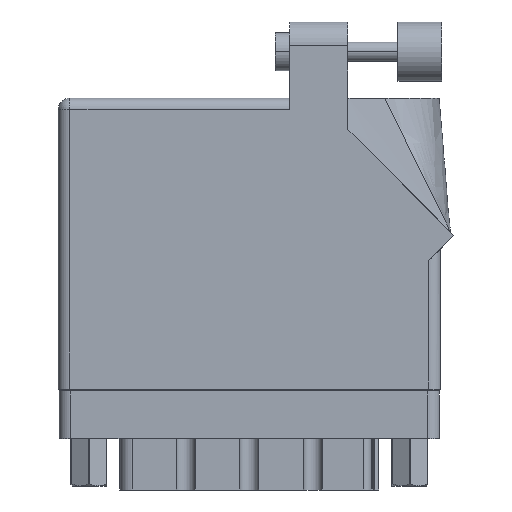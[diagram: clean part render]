
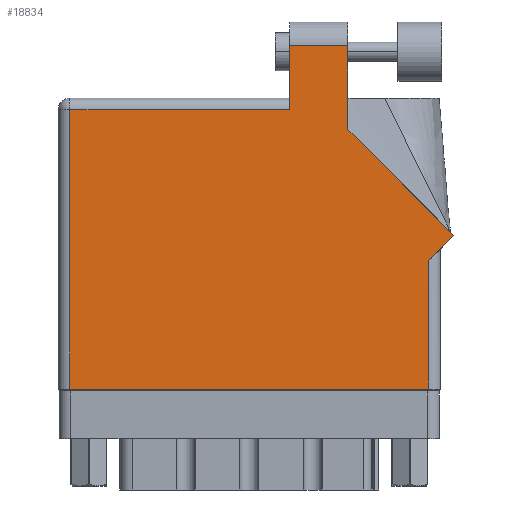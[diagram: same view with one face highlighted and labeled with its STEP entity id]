
A CAD part, front view. The second image highlights one B-rep face of the part: STEP entity #18834.
In plain terms, the highlighted face is planar.
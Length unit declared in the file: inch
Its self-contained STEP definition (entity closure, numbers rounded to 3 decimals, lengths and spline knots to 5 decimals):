
#185 = CARTESIAN_POINT ( 'NONE',  ( 0.062, 1.468, 0. ) ) ;
#529 = CARTESIAN_POINT ( 'NONE',  ( 1.524, 1.36442, 0. ) ) ;
#2475 = EDGE_CURVE ( 'NONE', #21599, #13160, #9164, .T. ) ;
#2711 = DIRECTION ( 'NONE',  ( 0., -1., 0. ) ) ;
#2892 = LINE ( 'NONE', #22346, #11988 ) ;
#3526 = CARTESIAN_POINT ( 'NONE',  ( 0.062, 0., 0. ) ) ;
#4853 = ORIENTED_EDGE ( 'NONE', *, *, #49832, .T. ) ;
#5081 = LINE ( 'NONE', #19882, #40089 ) ;
#5888 = CARTESIAN_POINT ( 'NONE',  ( 1.948, 0., 0. ) ) ;
#7686 = DIRECTION ( 'NONE',  ( 0., 0., -1. ) ) ;
#7887 = CARTESIAN_POINT ( 'NONE',  ( 1.948, 0.737, 0. ) ) ;
#7978 = VERTEX_POINT ( 'NONE', #42189 ) ;
#8332 = ORIENTED_EDGE ( 'NONE', *, *, #29546, .T. ) ;
#9164 = LINE ( 'NONE', #31423, #41724 ) ;
#9362 = LINE ( 'NONE', #35541, #27454 ) ;
#10418 = AXIS2_PLACEMENT_3D ( 'NONE', #46684, #7686, #23366 ) ;
#11100 = ORIENTED_EDGE ( 'NONE', *, *, #23640, .T. ) ;
#11988 = VECTOR ( 'NONE', #2711, 39.37008 ) ;
#12071 = DIRECTION ( 'NONE',  ( 0., -1., 0. ) ) ;
#12095 = CARTESIAN_POINT ( 'NONE',  ( 1.217, 1.805, 0. ) ) ;
#12140 = DIRECTION ( 'NONE',  ( 0.707, 0.707, 0. ) ) ;
#12303 = DIRECTION ( 'NONE',  ( 0., 1., 0. ) ) ;
#13160 = VERTEX_POINT ( 'NONE', #3526 ) ;
#13547 = ORIENTED_EDGE ( 'NONE', *, *, #33288, .T. ) ;
#13763 = VECTOR ( 'NONE', #20716, 39.37008 ) ;
#14477 = VERTEX_POINT ( 'NONE', #38979 ) ;
#14538 = FACE_OUTER_BOUND ( 'NONE', #25998, .T. ) ;
#14800 = VERTEX_POINT ( 'NONE', #25847 ) ;
#16198 = ORIENTED_EDGE ( 'NONE', *, *, #37717, .T. ) ;
#16261 = LINE ( 'NONE', #12095, #19901 ) ;
#18834 = ADVANCED_FACE ( 'NONE', ( #14538 ), #42511, .F. ) ;
#18990 = CARTESIAN_POINT ( 'NONE',  ( 2.08071, 0.80771, 0. ) ) ;
#19057 = DIRECTION ( 'NONE',  ( -1., 0., 0. ) ) ;
#19882 = CARTESIAN_POINT ( 'NONE',  ( 0., 1.468, 0. ) ) ;
#19901 = VECTOR ( 'NONE', #19057, 39.37008 ) ;
#20716 = DIRECTION ( 'NONE',  ( 0., 1., 0. ) ) ;
#21599 = VERTEX_POINT ( 'NONE', #185 ) ;
#22231 = LINE ( 'NONE', #44333, #13763 ) ;
#22346 = CARTESIAN_POINT ( 'NONE',  ( 1.217, 1.53, 0. ) ) ;
#23366 = DIRECTION ( 'NONE',  ( -1., 0., 0. ) ) ;
#23640 = EDGE_CURVE ( 'NONE', #33183, #21599, #5081, .T. ) ;
#23658 = ORIENTED_EDGE ( 'NONE', *, *, #2475, .T. ) ;
#23782 = DIRECTION ( 'NONE',  ( 1., 0., 0. ) ) ;
#24541 = LINE ( 'NONE', #18990, #48590 ) ;
#25847 = CARTESIAN_POINT ( 'NONE',  ( 1.524, 1.805, 0. ) ) ;
#25998 = EDGE_LOOP ( 'NONE', ( #4853, #31379, #16198, #11100, #23658, #13547, #8332, #40610, #35403 ) ) ;
#26189 = VECTOR ( 'NONE', #12303, 39.37008 ) ;
#26831 = CARTESIAN_POINT ( 'NONE',  ( 1.217, 1.468, 0. ) ) ;
#27454 = VECTOR ( 'NONE', #12140, 39.37008 ) ;
#27511 = EDGE_CURVE ( 'NONE', #14477, #28254, #24541, .T. ) ;
#27659 = CARTESIAN_POINT ( 'NONE',  ( 0., 0., 0. ) ) ;
#28254 = VERTEX_POINT ( 'NONE', #529 ) ;
#29218 = VERTEX_POINT ( 'NONE', #48445 ) ;
#29546 = EDGE_CURVE ( 'NONE', #40837, #7978, #38210, .T. ) ;
#31379 = ORIENTED_EDGE ( 'NONE', *, *, #49606, .T. ) ;
#31423 = CARTESIAN_POINT ( 'NONE',  ( 0.062, 0., 0. ) ) ;
#33183 = VERTEX_POINT ( 'NONE', #26831 ) ;
#33288 = EDGE_CURVE ( 'NONE', #13160, #40837, #42119, .T. ) ;
#35403 = ORIENTED_EDGE ( 'NONE', *, *, #27511, .T. ) ;
#35541 = CARTESIAN_POINT ( 'NONE',  ( 2.01, 0.737, 0. ) ) ;
#37717 = EDGE_CURVE ( 'NONE', #29218, #33183, #2892, .T. ) ;
#37878 = VECTOR ( 'NONE', #23782, 39.37008 ) ;
#38210 = LINE ( 'NONE', #7887, #26189 ) ;
#38979 = CARTESIAN_POINT ( 'NONE',  ( 2.08071, 0.80771, 0. ) ) ;
#40089 = VECTOR ( 'NONE', #43354, 39.37008 ) ;
#40610 = ORIENTED_EDGE ( 'NONE', *, *, #41158, .T. ) ;
#40837 = VERTEX_POINT ( 'NONE', #5888 ) ;
#41158 = EDGE_CURVE ( 'NONE', #7978, #14477, #9362, .T. ) ;
#41724 = VECTOR ( 'NONE', #12071, 39.37008 ) ;
#42119 = LINE ( 'NONE', #27659, #37878 ) ;
#42189 = CARTESIAN_POINT ( 'NONE',  ( 1.948, 0.675, 0. ) ) ;
#42471 = DIRECTION ( 'NONE',  ( -0.707, 0.707, 0. ) ) ;
#42511 = PLANE ( 'NONE',  #10418 ) ;
#43354 = DIRECTION ( 'NONE',  ( -1., 0., 0. ) ) ;
#44333 = CARTESIAN_POINT ( 'NONE',  ( 1.524, 1.36442, 0. ) ) ;
#46684 = CARTESIAN_POINT ( 'NONE',  ( 0., 1.53, 0. ) ) ;
#48445 = CARTESIAN_POINT ( 'NONE',  ( 1.217, 1.805, 0. ) ) ;
#48590 = VECTOR ( 'NONE', #42471, 39.37008 ) ;
#49606 = EDGE_CURVE ( 'NONE', #14800, #29218, #16261, .T. ) ;
#49832 = EDGE_CURVE ( 'NONE', #28254, #14800, #22231, .T. ) ;
